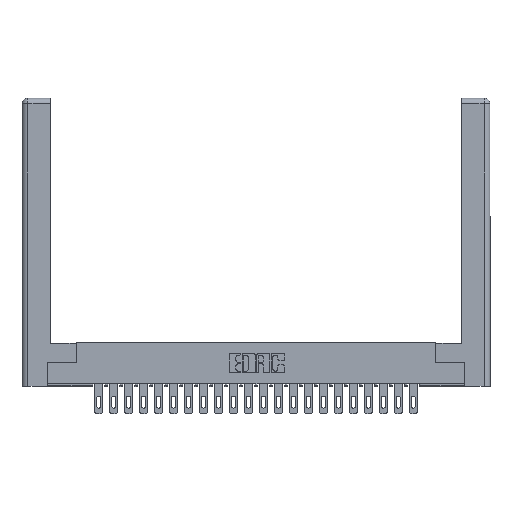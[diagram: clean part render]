
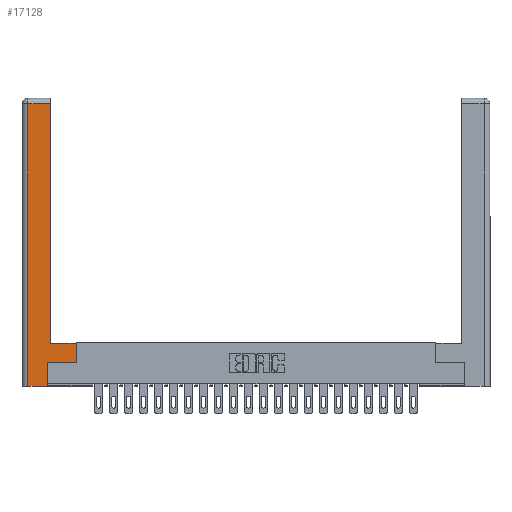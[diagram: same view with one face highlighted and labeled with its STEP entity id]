
A CAD part, top view. The second image highlights one B-rep face of the part: STEP entity #17128.
In plain terms, the highlighted planar face has unit normal (0, 0, 1).
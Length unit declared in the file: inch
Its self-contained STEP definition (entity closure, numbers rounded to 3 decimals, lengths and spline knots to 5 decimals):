
#289 = VERTEX_POINT ( 'NONE', #13843 ) ;
#1137 = LINE ( 'NONE', #23420, #25941 ) ;
#1203 = EDGE_LOOP ( 'NONE', ( #25828, #12752, #17959, #21843, #5438, #17165, #8505, #5178 ) ) ;
#1738 = EDGE_CURVE ( 'NONE', #20264, #14961, #17166, .T. ) ;
#2093 = LINE ( 'NONE', #3711, #9756 ) ;
#2488 = CARTESIAN_POINT ( 'NONE',  ( 0.295, 0.45, 0. ) ) ;
#2757 = VERTEX_POINT ( 'NONE', #19435 ) ;
#3711 = CARTESIAN_POINT ( 'NONE',  ( 0.0615, 2.94, 0. ) ) ;
#4879 = DIRECTION ( 'NONE',  ( 1., 0., 0. ) ) ;
#5178 = ORIENTED_EDGE ( 'NONE', *, *, #24152, .T. ) ;
#5351 = VERTEX_POINT ( 'NONE', #15734 ) ;
#5438 = ORIENTED_EDGE ( 'NONE', *, *, #21083, .T. ) ;
#5557 = EDGE_CURVE ( 'NONE', #15182, #2757, #18316, .T. ) ;
#5768 = CARTESIAN_POINT ( 'NONE',  ( 0.0615, 0., 0. ) ) ;
#6281 = CARTESIAN_POINT ( 'NONE',  ( 0., 0., 0. ) ) ;
#6439 = CARTESIAN_POINT ( 'NONE',  ( 0.265, 0.245, 0. ) ) ;
#6780 = DIRECTION ( 'NONE',  ( 1., 0., 0. ) ) ;
#7014 = CARTESIAN_POINT ( 'NONE',  ( 0.565, 0.245, 0. ) ) ;
#8319 = PLANE ( 'NONE',  #23485 ) ;
#8505 = ORIENTED_EDGE ( 'NONE', *, *, #14808, .T. ) ;
#9738 = LINE ( 'NONE', #12858, #11152 ) ;
#9756 = VECTOR ( 'NONE', #10996, 39.37008 ) ;
#10025 = LINE ( 'NONE', #28764, #27178 ) ;
#10314 = EDGE_CURVE ( 'NONE', #5351, #25421, #2093, .T. ) ;
#10673 = DIRECTION ( 'NONE',  ( 0., 1., 0. ) ) ;
#10996 = DIRECTION ( 'NONE',  ( -1., 0., 0. ) ) ;
#11152 = VECTOR ( 'NONE', #10673, 39.37008 ) ;
#11372 = CARTESIAN_POINT ( 'NONE',  ( 0.565, 0.245, 0. ) ) ;
#12752 = ORIENTED_EDGE ( 'NONE', *, *, #10314, .T. ) ;
#12858 = CARTESIAN_POINT ( 'NONE',  ( 0.265, 0.245, 0. ) ) ;
#13843 = CARTESIAN_POINT ( 'NONE',  ( 0.565, 0.45, 0. ) ) ;
#14018 = DIRECTION ( 'NONE',  ( -1., 0., 0. ) ) ;
#14227 = DIRECTION ( 'NONE',  ( 0., 1., 0. ) ) ;
#14377 = DIRECTION ( 'NONE',  ( 0., -1., 0. ) ) ;
#14808 = EDGE_CURVE ( 'NONE', #14961, #289, #10025, .T. ) ;
#14961 = VERTEX_POINT ( 'NONE', #11372 ) ;
#15182 = VERTEX_POINT ( 'NONE', #5768 ) ;
#15279 = VECTOR ( 'NONE', #14377, 39.37008 ) ;
#15517 = VECTOR ( 'NONE', #14018, 39.37008 ) ;
#15734 = CARTESIAN_POINT ( 'NONE',  ( 0.295, 2.94, 0. ) ) ;
#17128 = ADVANCED_FACE ( 'NONE', ( #23213 ), #8319, .F. ) ;
#17165 = ORIENTED_EDGE ( 'NONE', *, *, #1738, .T. ) ;
#17166 = LINE ( 'NONE', #7014, #25241 ) ;
#17333 = CARTESIAN_POINT ( 'NONE',  ( 0.0615, 2.94, 0. ) ) ;
#17959 = ORIENTED_EDGE ( 'NONE', *, *, #22105, .T. ) ;
#18316 = LINE ( 'NONE', #26825, #18677 ) ;
#18677 = VECTOR ( 'NONE', #6780, 39.37008 ) ;
#19365 = EDGE_CURVE ( 'NONE', #19667, #5351, #1137, .T. ) ;
#19435 = CARTESIAN_POINT ( 'NONE',  ( 0.265, 0., 0. ) ) ;
#19576 = DIRECTION ( 'NONE',  ( -1., 0., 0. ) ) ;
#19661 = DIRECTION ( 'NONE',  ( 0., 0., -1. ) ) ;
#19667 = VERTEX_POINT ( 'NONE', #2488 ) ;
#20264 = VERTEX_POINT ( 'NONE', #6439 ) ;
#21083 = EDGE_CURVE ( 'NONE', #2757, #20264, #9738, .T. ) ;
#21843 = ORIENTED_EDGE ( 'NONE', *, *, #5557, .T. ) ;
#22105 = EDGE_CURVE ( 'NONE', #25421, #15182, #23349, .T. ) ;
#23039 = CARTESIAN_POINT ( 'NONE',  ( 0.295, 0.45, 0. ) ) ;
#23213 = FACE_OUTER_BOUND ( 'NONE', #1203, .T. ) ;
#23279 = CARTESIAN_POINT ( 'NONE',  ( 0.0615, 0., 0. ) ) ;
#23349 = LINE ( 'NONE', #23279, #15279 ) ;
#23420 = CARTESIAN_POINT ( 'NONE',  ( 0.295, 3., 0. ) ) ;
#23485 = AXIS2_PLACEMENT_3D ( 'NONE', #6281, #19661, #19576 ) ;
#23968 = LINE ( 'NONE', #23039, #15517 ) ;
#24152 = EDGE_CURVE ( 'NONE', #289, #19667, #23968, .T. ) ;
#24302 = DIRECTION ( 'NONE',  ( 0., 1., 0. ) ) ;
#25241 = VECTOR ( 'NONE', #4879, 39.37008 ) ;
#25421 = VERTEX_POINT ( 'NONE', #17333 ) ;
#25828 = ORIENTED_EDGE ( 'NONE', *, *, #19365, .T. ) ;
#25941 = VECTOR ( 'NONE', #14227, 39.37008 ) ;
#26825 = CARTESIAN_POINT ( 'NONE',  ( 0.265, 0., 0. ) ) ;
#27178 = VECTOR ( 'NONE', #24302, 39.37008 ) ;
#28764 = CARTESIAN_POINT ( 'NONE',  ( 0.565, 0.45, 0. ) ) ;
